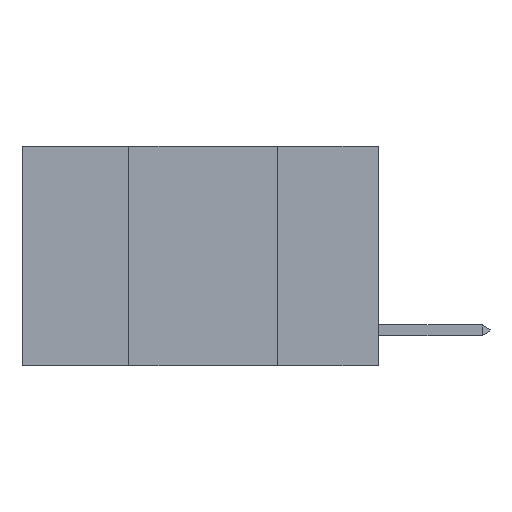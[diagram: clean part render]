
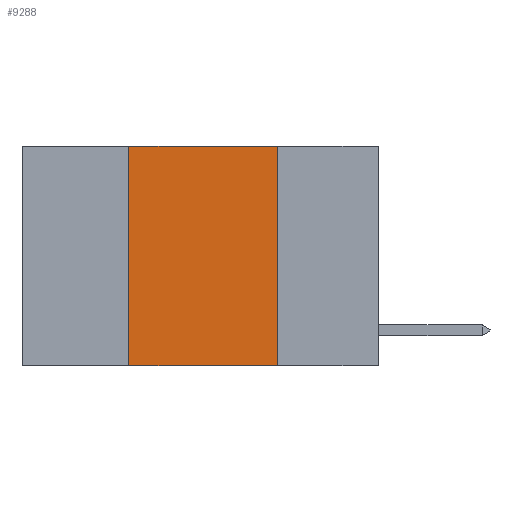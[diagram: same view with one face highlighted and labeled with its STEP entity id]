
A CAD part, left-side view. The second image highlights one B-rep face of the part: STEP entity #9288.
In plain terms, the highlighted planar face has unit normal (-1, 0, 0).
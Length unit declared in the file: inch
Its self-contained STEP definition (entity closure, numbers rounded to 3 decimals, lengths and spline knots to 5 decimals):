
#60 = EDGE_CURVE ( 'NONE', #13207, #5227, #17538, .T. ) ;
#408 = CARTESIAN_POINT ( 'NONE',  ( 0., 0.17, 0. ) ) ;
#867 = EDGE_LOOP ( 'NONE', ( #14672, #17965, #2973, #10361 ) ) ;
#1417 = DIRECTION ( 'NONE',  ( 0., -1., 0. ) ) ;
#1679 = DIRECTION ( 'NONE',  ( 0., 0., 1. ) ) ;
#1790 = LINE ( 'NONE', #408, #7738 ) ;
#2973 = ORIENTED_EDGE ( 'NONE', *, *, #6607, .F. ) ;
#3071 = FACE_OUTER_BOUND ( 'NONE', #867, .T. ) ;
#3321 = CARTESIAN_POINT ( 'NONE',  ( 0., 0.42, 0. ) ) ;
#3744 = VERTEX_POINT ( 'NONE', #6770 ) ;
#4246 = CARTESIAN_POINT ( 'NONE',  ( 0., 0.6, 0. ) ) ;
#5190 = DIRECTION ( 'NONE',  ( 0., -1., 0. ) ) ;
#5227 = VERTEX_POINT ( 'NONE', #14088 ) ;
#5817 = DIRECTION ( 'NONE',  ( 0., 0., -1. ) ) ;
#6489 = CARTESIAN_POINT ( 'NONE',  ( 0., 0.6, -0.37 ) ) ;
#6607 = EDGE_CURVE ( 'NONE', #13207, #16292, #17813, .T. ) ;
#6770 = CARTESIAN_POINT ( 'NONE',  ( 0., 0.17, 0. ) ) ;
#7738 = VECTOR ( 'NONE', #15316, 39.37008 ) ;
#8116 = LINE ( 'NONE', #4246, #15783 ) ;
#8380 = VECTOR ( 'NONE', #5190, 39.37008 ) ;
#9288 = ADVANCED_FACE ( 'NONE', ( #3071 ), #15779, .F. ) ;
#9586 = EDGE_CURVE ( 'NONE', #16292, #3744, #8116, .T. ) ;
#10361 = ORIENTED_EDGE ( 'NONE', *, *, #60, .T. ) ;
#12657 = CARTESIAN_POINT ( 'NONE',  ( 0., 0.42, 0. ) ) ;
#12945 = DIRECTION ( 'NONE',  ( 1., 0., 0. ) ) ;
#13199 = AXIS2_PLACEMENT_3D ( 'NONE', #17322, #12945, #5817 ) ;
#13207 = VERTEX_POINT ( 'NONE', #13769 ) ;
#13769 = CARTESIAN_POINT ( 'NONE',  ( 0., 0.42, -0.37 ) ) ;
#14088 = CARTESIAN_POINT ( 'NONE',  ( 0., 0.17, -0.37 ) ) ;
#14167 = VECTOR ( 'NONE', #1679, 39.37008 ) ;
#14340 = EDGE_CURVE ( 'NONE', #3744, #5227, #1790, .T. ) ;
#14672 = ORIENTED_EDGE ( 'NONE', *, *, #14340, .F. ) ;
#15316 = DIRECTION ( 'NONE',  ( 0., 0., -1. ) ) ;
#15779 = PLANE ( 'NONE',  #13199 ) ;
#15783 = VECTOR ( 'NONE', #1417, 39.37008 ) ;
#16292 = VERTEX_POINT ( 'NONE', #3321 ) ;
#17322 = CARTESIAN_POINT ( 'NONE',  ( 0., 0.6, 0. ) ) ;
#17538 = LINE ( 'NONE', #6489, #8380 ) ;
#17813 = LINE ( 'NONE', #12657, #14167 ) ;
#17965 = ORIENTED_EDGE ( 'NONE', *, *, #9586, .F. ) ;
